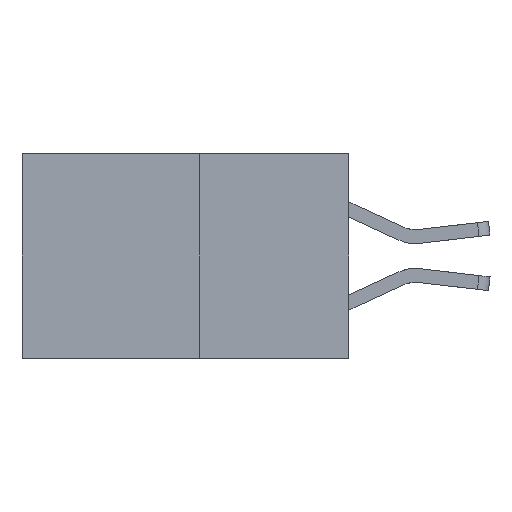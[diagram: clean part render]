
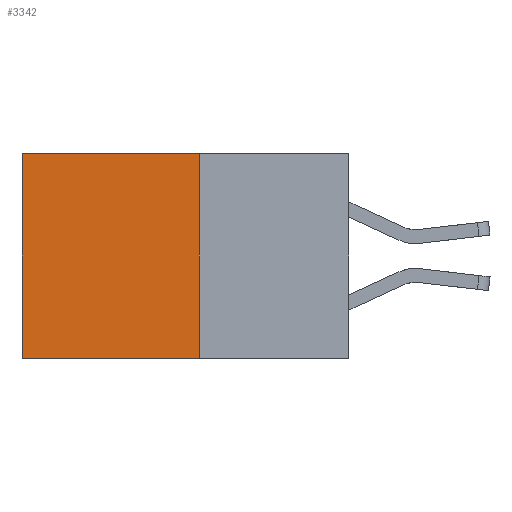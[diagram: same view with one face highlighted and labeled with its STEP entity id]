
A CAD part, left-side view. The second image highlights one B-rep face of the part: STEP entity #3342.
In plain terms, the highlighted planar face has unit normal (-1, 0, 0).
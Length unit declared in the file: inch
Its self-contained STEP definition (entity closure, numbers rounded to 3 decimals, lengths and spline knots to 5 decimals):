
#257 = FACE_OUTER_BOUND ( 'NONE', #10054, .T. ) ;
#382 = CARTESIAN_POINT ( 'NONE',  ( 0.277, 0.27, 0. ) ) ;
#569 = AXIS2_PLACEMENT_3D ( 'NONE', #6621, #5818, #7190 ) ;
#839 = DIRECTION ( 'NONE',  ( 0., 1., 0. ) ) ;
#877 = EDGE_CURVE ( 'NONE', #7272, #4420, #7511, .T. ) ;
#1232 = VECTOR ( 'NONE', #7843, 39.37008 ) ;
#2040 = EDGE_CURVE ( 'NONE', #3969, #4420, #3741, .T. ) ;
#2277 = EDGE_CURVE ( 'NONE', #8680, #3969, #4827, .T. ) ;
#2654 = VECTOR ( 'NONE', #5073, 39.37008 ) ;
#2862 = EDGE_CURVE ( 'NONE', #8680, #7272, #9563, .T. ) ;
#3077 = CARTESIAN_POINT ( 'NONE',  ( 0.277, 0.27, -0.37 ) ) ;
#3342 = ADVANCED_FACE ( 'NONE', ( #257 ), #6557, .F. ) ;
#3741 = LINE ( 'NONE', #9038, #1232 ) ;
#3969 = VERTEX_POINT ( 'NONE', #5554 ) ;
#4240 = VECTOR ( 'NONE', #8730, 39.37008 ) ;
#4272 = CARTESIAN_POINT ( 'NONE',  ( 0.277, 0.27, 0. ) ) ;
#4420 = VERTEX_POINT ( 'NONE', #8127 ) ;
#4827 = LINE ( 'NONE', #382, #2654 ) ;
#5073 = DIRECTION ( 'NONE',  ( 0., 1., 0. ) ) ;
#5485 = ORIENTED_EDGE ( 'NONE', *, *, #2040, .T. ) ;
#5537 = ORIENTED_EDGE ( 'NONE', *, *, #877, .F. ) ;
#5552 = ORIENTED_EDGE ( 'NONE', *, *, #2862, .F. ) ;
#5554 = CARTESIAN_POINT ( 'NONE',  ( 0.277, 0.59, 0. ) ) ;
#5603 = ORIENTED_EDGE ( 'NONE', *, *, #2277, .T. ) ;
#5818 = DIRECTION ( 'NONE',  ( 1., 0., 0. ) ) ;
#6557 = PLANE ( 'NONE',  #569 ) ;
#6621 = CARTESIAN_POINT ( 'NONE',  ( 0.277, 0.27, -0.37 ) ) ;
#7190 = DIRECTION ( 'NONE',  ( 0., 0., -1. ) ) ;
#7272 = VERTEX_POINT ( 'NONE', #3077 ) ;
#7422 = CARTESIAN_POINT ( 'NONE',  ( 0.277, 0.27, -0.37 ) ) ;
#7511 = LINE ( 'NONE', #7422, #9350 ) ;
#7843 = DIRECTION ( 'NONE',  ( 0., 0., -1. ) ) ;
#8127 = CARTESIAN_POINT ( 'NONE',  ( 0.277, 0.59, -0.37 ) ) ;
#8680 = VERTEX_POINT ( 'NONE', #4272 ) ;
#8730 = DIRECTION ( 'NONE',  ( 0., 0., -1. ) ) ;
#9038 = CARTESIAN_POINT ( 'NONE',  ( 0.277, 0.59, -0.37 ) ) ;
#9350 = VECTOR ( 'NONE', #839, 39.37008 ) ;
#9563 = LINE ( 'NONE', #9866, #4240 ) ;
#9866 = CARTESIAN_POINT ( 'NONE',  ( 0.277, 0.27, -0.37 ) ) ;
#10054 = EDGE_LOOP ( 'NONE', ( #5485, #5537, #5552, #5603 ) ) ;
